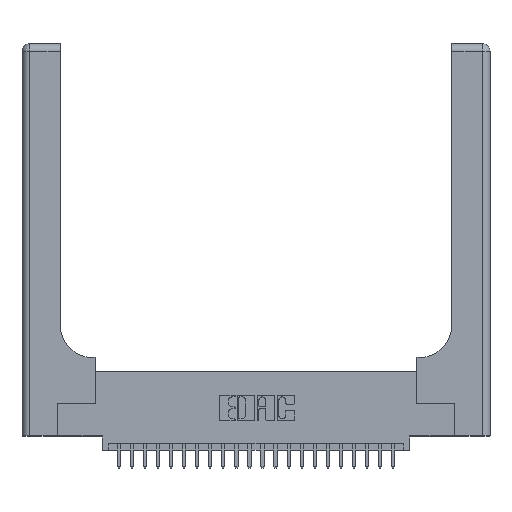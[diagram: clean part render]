
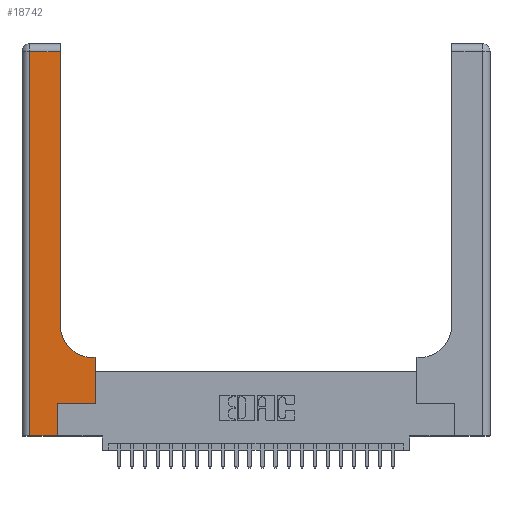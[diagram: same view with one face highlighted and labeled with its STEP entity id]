
A CAD part, top view. The second image highlights one B-rep face of the part: STEP entity #18742.
In plain terms, the highlighted planar face has unit normal (0, 0, 1).
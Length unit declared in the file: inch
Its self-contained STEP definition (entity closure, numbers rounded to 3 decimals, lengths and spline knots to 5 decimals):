
#232 = VECTOR ( 'NONE', #19819, 39.37008 ) ;
#667 = ORIENTED_EDGE ( 'NONE', *, *, #19987, .T. ) ;
#934 = EDGE_CURVE ( 'NONE', #21020, #1145, #17425, .T. ) ;
#1120 = DIRECTION ( 'NONE',  ( 0., -1., 0. ) ) ;
#1145 = VERTEX_POINT ( 'NONE', #7966 ) ;
#1158 = EDGE_CURVE ( 'NONE', #2268, #19004, #22858, .T. ) ;
#1536 = DIRECTION ( 'NONE',  ( 0., 1., 0. ) ) ;
#1808 = VECTOR ( 'NONE', #7266, 39.37008 ) ;
#1897 = CARTESIAN_POINT ( 'NONE',  ( 0.2915, 3., 0.37 ) ) ;
#2116 = CARTESIAN_POINT ( 'NONE',  ( 0.269, 0.25, 0.37 ) ) ;
#2199 = CARTESIAN_POINT ( 'NONE',  ( 0.269, 0., 0.37 ) ) ;
#2205 = AXIS2_PLACEMENT_3D ( 'NONE', #3573, #5660, #19173 ) ;
#2262 = ORIENTED_EDGE ( 'NONE', *, *, #2632, .T. ) ;
#2268 = VERTEX_POINT ( 'NONE', #12992 ) ;
#2632 = EDGE_CURVE ( 'NONE', #1145, #4467, #24754, .T. ) ;
#3573 = CARTESIAN_POINT ( 'NONE',  ( 0., 3., 0.37 ) ) ;
#3702 = EDGE_CURVE ( 'NONE', #4949, #2268, #17709, .T. ) ;
#3803 = DIRECTION ( 'NONE',  ( 1., 0., 0. ) ) ;
#4215 = LINE ( 'NONE', #1897, #9473 ) ;
#4467 = VERTEX_POINT ( 'NONE', #22329 ) ;
#4949 = VERTEX_POINT ( 'NONE', #21812 ) ;
#5660 = DIRECTION ( 'NONE',  ( 0., 0., -1. ) ) ;
#6608 = CARTESIAN_POINT ( 'NONE',  ( 0.06, 0., 0.37 ) ) ;
#7266 = DIRECTION ( 'NONE',  ( 0., 1., 0. ) ) ;
#7473 = ORIENTED_EDGE ( 'NONE', *, *, #24043, .T. ) ;
#7830 = ORIENTED_EDGE ( 'NONE', *, *, #934, .T. ) ;
#7956 = ORIENTED_EDGE ( 'NONE', *, *, #11638, .T. ) ;
#7966 = CARTESIAN_POINT ( 'NONE',  ( 0.269, 0.25, 0.37 ) ) ;
#8085 = LINE ( 'NONE', #11710, #13223 ) ;
#8153 = DIRECTION ( 'NONE',  ( 1., 0., 0. ) ) ;
#8512 = CARTESIAN_POINT ( 'NONE',  ( 0.5415, 0.85, 0.37 ) ) ;
#9379 = EDGE_CURVE ( 'NONE', #12513, #20446, #18349, .T. ) ;
#9473 = VECTOR ( 'NONE', #16946, 39.37008 ) ;
#10466 = DIRECTION ( 'NONE',  ( 1., 0., 0. ) ) ;
#10777 = LINE ( 'NONE', #17879, #232 ) ;
#11638 = EDGE_CURVE ( 'NONE', #17772, #12513, #10777, .T. ) ;
#11710 = CARTESIAN_POINT ( 'NONE',  ( 0., 0., 0.37 ) ) ;
#11768 = ORIENTED_EDGE ( 'NONE', *, *, #3702, .T. ) ;
#12028 = VECTOR ( 'NONE', #16228, 39.37008 ) ;
#12266 = AXIS2_PLACEMENT_3D ( 'NONE', #8512, #21991, #10466 ) ;
#12327 = VECTOR ( 'NONE', #1536, 39.37008 ) ;
#12513 = VERTEX_POINT ( 'NONE', #24966 ) ;
#12533 = ORIENTED_EDGE ( 'NONE', *, *, #17546, .T. ) ;
#12992 = CARTESIAN_POINT ( 'NONE',  ( 0.06, 2.94, 0.37 ) ) ;
#13117 = CARTESIAN_POINT ( 'NONE',  ( 0.5585, 0.25, 0.37 ) ) ;
#13223 = VECTOR ( 'NONE', #3803, 39.37008 ) ;
#16076 = CARTESIAN_POINT ( 'NONE',  ( 0., 2.94, 0.37 ) ) ;
#16228 = DIRECTION ( 'NONE',  ( -1., 0., 0. ) ) ;
#16309 = CARTESIAN_POINT ( 'NONE',  ( 0.5585, 0.6, 0.37 ) ) ;
#16946 = DIRECTION ( 'NONE',  ( 0., 1., 0. ) ) ;
#17261 = PLANE ( 'NONE',  #2205 ) ;
#17353 = ORIENTED_EDGE ( 'NONE', *, *, #9379, .T. ) ;
#17425 = LINE ( 'NONE', #2199, #12327 ) ;
#17546 = EDGE_CURVE ( 'NONE', #19004, #21020, #8085, .T. ) ;
#17709 = LINE ( 'NONE', #16076, #12028 ) ;
#17772 = VERTEX_POINT ( 'NONE', #16309 ) ;
#17879 = CARTESIAN_POINT ( 'NONE',  ( 0.2915, 0.6, 0.37 ) ) ;
#17886 = CARTESIAN_POINT ( 'NONE',  ( 0.06, 3., 0.37 ) ) ;
#18005 = LINE ( 'NONE', #13117, #1808 ) ;
#18158 = EDGE_LOOP ( 'NONE', ( #667, #11768, #20088, #12533, #7830, #2262, #7473, #7956, #17353 ) ) ;
#18297 = VECTOR ( 'NONE', #1120, 39.37008 ) ;
#18349 = CIRCLE ( 'NONE', #12266, 0.25 ) ;
#18742 = ADVANCED_FACE ( 'NONE', ( #21895 ), #17261, .F. ) ;
#19004 = VERTEX_POINT ( 'NONE', #6608 ) ;
#19173 = DIRECTION ( 'NONE',  ( -1., 0., 0. ) ) ;
#19567 = VECTOR ( 'NONE', #8153, 39.37008 ) ;
#19819 = DIRECTION ( 'NONE',  ( -1., 0., 0. ) ) ;
#19987 = EDGE_CURVE ( 'NONE', #20446, #4949, #4215, .T. ) ;
#20088 = ORIENTED_EDGE ( 'NONE', *, *, #1158, .T. ) ;
#20446 = VERTEX_POINT ( 'NONE', #21164 ) ;
#21020 = VERTEX_POINT ( 'NONE', #24872 ) ;
#21164 = CARTESIAN_POINT ( 'NONE',  ( 0.2915, 0.85, 0.37 ) ) ;
#21812 = CARTESIAN_POINT ( 'NONE',  ( 0.2915, 2.94, 0.37 ) ) ;
#21895 = FACE_OUTER_BOUND ( 'NONE', #18158, .T. ) ;
#21991 = DIRECTION ( 'NONE',  ( 0., 0., -1. ) ) ;
#22329 = CARTESIAN_POINT ( 'NONE',  ( 0.5585, 0.25, 0.37 ) ) ;
#22858 = LINE ( 'NONE', #17886, #18297 ) ;
#24043 = EDGE_CURVE ( 'NONE', #4467, #17772, #18005, .T. ) ;
#24754 = LINE ( 'NONE', #2116, #19567 ) ;
#24872 = CARTESIAN_POINT ( 'NONE',  ( 0.269, 0., 0.37 ) ) ;
#24966 = CARTESIAN_POINT ( 'NONE',  ( 0.5415, 0.6, 0.37 ) ) ;
